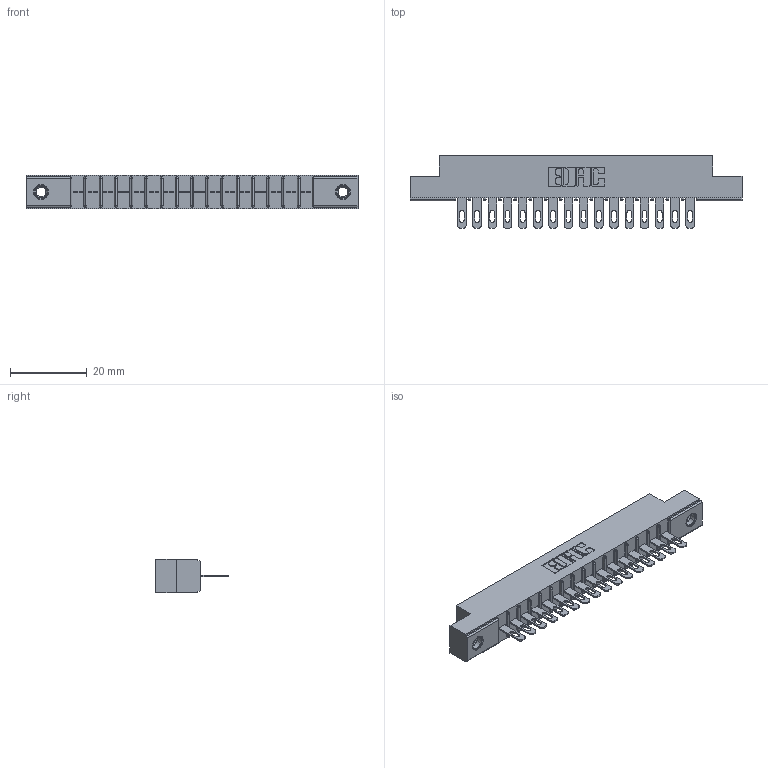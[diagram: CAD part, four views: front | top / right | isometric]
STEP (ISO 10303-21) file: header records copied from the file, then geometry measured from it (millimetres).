
FILE_DESCRIPTION (( 'STEP AP203' ), '1' );
FILE_NAME ('356-016-400-107.STEP', '2020-09-23T12:25:31', ( '' ), ( '' ), 'SwSTEP 2.0', 'SolidWorks 2020', '' );
FILE_SCHEMA (( 'CONFIG_CONTROL_DESIGN' ));
Length unit declared in the file: inch
Products named in the file (4): 345-250-001_345-250-005-103; 356-016-400-107; 306-290-001_100; 306 Part_.156 Dia
Assembly tree (19 placements, depth 2):
  356-016-400-107
    306 Part_.156 Dia
    306-290-001_100  x16
    345-250-001_345-250-005-103  x2
Bounding box: 86.41 x 18.87 x 8.71 mm (x, y, z)
Volume: 5917.3 mm3; surface area: 8862.9 mm2
Topology: 19 solids, 19 shells, 1392 faces, 3892 edges, 2500 vertices
Faces by surface type: plane 900, cylinder 412, sphere 64, cone 12, torus 4
Entity records: 19638 total; most frequent: CARTESIAN_POINT 3274, DIRECTION 3240, ORIENTED_EDGE 3236, EDGE_CURVE 1618, LINE 1248, VECTOR 1248, VERTEX_POINT 1030, AXIS2_PLACEMENT_3D 996
